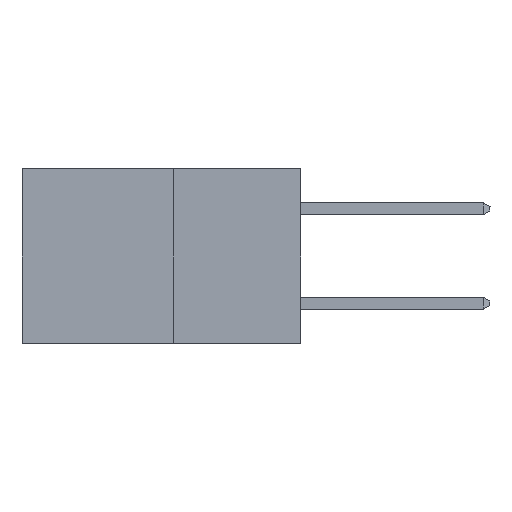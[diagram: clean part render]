
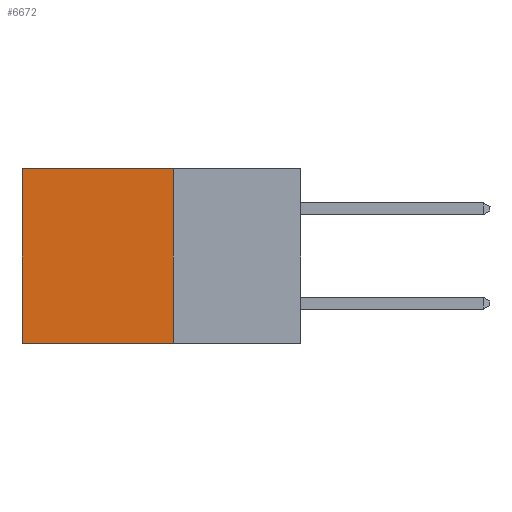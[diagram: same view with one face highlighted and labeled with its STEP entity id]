
A CAD part, left-side view. The second image highlights one B-rep face of the part: STEP entity #6672.
In plain terms, the highlighted planar face has unit normal (-1, 0, 0).
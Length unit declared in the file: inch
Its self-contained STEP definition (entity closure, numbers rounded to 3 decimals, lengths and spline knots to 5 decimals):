
#645 = DIRECTION ( 'NONE',  ( 0., 1., 0. ) ) ;
#853 = VECTOR ( 'NONE', #5244, 39.37008 ) ;
#1007 = VERTEX_POINT ( 'NONE', #2908 ) ;
#1257 = LINE ( 'NONE', #10237, #5352 ) ;
#1369 = VERTEX_POINT ( 'NONE', #3478 ) ;
#1513 = CARTESIAN_POINT ( 'NONE',  ( 0.277, 0.27, -0.37 ) ) ;
#1514 = ORIENTED_EDGE ( 'NONE', *, *, #9917, .T. ) ;
#1522 = CARTESIAN_POINT ( 'NONE',  ( 0.277, 0.59, -0.37 ) ) ;
#1752 = EDGE_CURVE ( 'NONE', #1369, #1007, #9421, .T. ) ;
#1794 = ORIENTED_EDGE ( 'NONE', *, *, #3893, .F. ) ;
#2389 = DIRECTION ( 'NONE',  ( 0., 0., -1. ) ) ;
#2485 = LINE ( 'NONE', #1522, #10259 ) ;
#2728 = FACE_OUTER_BOUND ( 'NONE', #8210, .T. ) ;
#2908 = CARTESIAN_POINT ( 'NONE',  ( 0.277, 0.59, -0.37 ) ) ;
#3478 = CARTESIAN_POINT ( 'NONE',  ( 0.277, 0.27, -0.37 ) ) ;
#3893 = EDGE_CURVE ( 'NONE', #5844, #1369, #4397, .T. ) ;
#3968 = ORIENTED_EDGE ( 'NONE', *, *, #8314, .T. ) ;
#4374 = AXIS2_PLACEMENT_3D ( 'NONE', #9735, #5120, #10453 ) ;
#4391 = CARTESIAN_POINT ( 'NONE',  ( 0.277, 0.59, 0. ) ) ;
#4397 = LINE ( 'NONE', #1513, #6269 ) ;
#5120 = DIRECTION ( 'NONE',  ( 1., 0., 0. ) ) ;
#5244 = DIRECTION ( 'NONE',  ( 0., 1., 0. ) ) ;
#5352 = VECTOR ( 'NONE', #645, 39.37008 ) ;
#5844 = VERTEX_POINT ( 'NONE', #9842 ) ;
#6015 = CARTESIAN_POINT ( 'NONE',  ( 0.277, 0.27, -0.37 ) ) ;
#6269 = VECTOR ( 'NONE', #2389, 39.37008 ) ;
#6672 = ADVANCED_FACE ( 'NONE', ( #2728 ), #8971, .F. ) ;
#7931 = ORIENTED_EDGE ( 'NONE', *, *, #1752, .F. ) ;
#7981 = DIRECTION ( 'NONE',  ( 0., 0., -1. ) ) ;
#8210 = EDGE_LOOP ( 'NONE', ( #1514, #7931, #1794, #3968 ) ) ;
#8314 = EDGE_CURVE ( 'NONE', #5844, #10480, #1257, .T. ) ;
#8971 = PLANE ( 'NONE',  #4374 ) ;
#9421 = LINE ( 'NONE', #6015, #853 ) ;
#9735 = CARTESIAN_POINT ( 'NONE',  ( 0.277, 0.27, -0.37 ) ) ;
#9842 = CARTESIAN_POINT ( 'NONE',  ( 0.277, 0.27, 0. ) ) ;
#9917 = EDGE_CURVE ( 'NONE', #10480, #1007, #2485, .T. ) ;
#10237 = CARTESIAN_POINT ( 'NONE',  ( 0.277, 0.27, 0. ) ) ;
#10259 = VECTOR ( 'NONE', #7981, 39.37008 ) ;
#10453 = DIRECTION ( 'NONE',  ( 0., 0., -1. ) ) ;
#10480 = VERTEX_POINT ( 'NONE', #4391 ) ;
